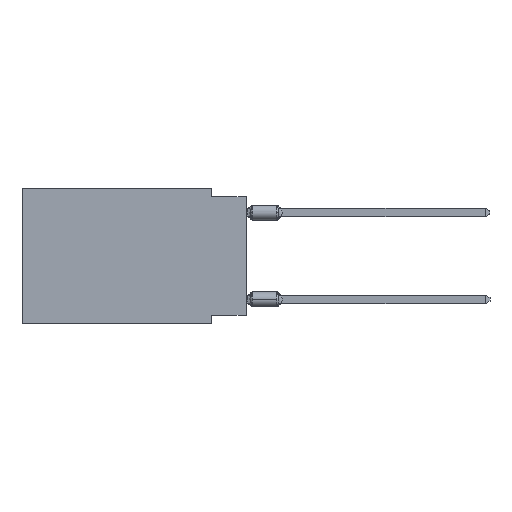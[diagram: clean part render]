
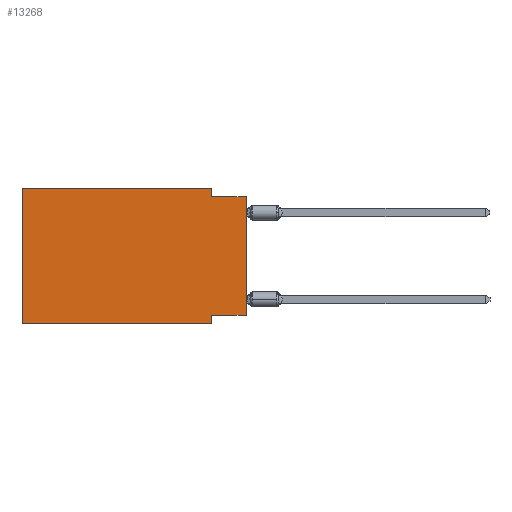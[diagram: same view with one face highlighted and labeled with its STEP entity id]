
A CAD part, left-side view. The second image highlights one B-rep face of the part: STEP entity #13268.
In plain terms, the highlighted planar face has unit normal (-1, 0, 0).
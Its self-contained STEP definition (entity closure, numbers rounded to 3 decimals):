
#137 = LINE ( 'NONE', #13860, #9160 ) ;
#380 = VERTEX_POINT ( 'NONE', #4488 ) ;
#620 = CARTESIAN_POINT ( 'NONE',  ( 0., 16.383, 0. ) ) ;
#703 = DIRECTION ( 'NONE',  ( 0., 0., -1. ) ) ;
#1499 = LINE ( 'NONE', #11670, #16042 ) ;
#1540 = EDGE_LOOP ( 'NONE', ( #11671, #7039, #22111, #13232, #17227, #22080, #11189, #18426 ) ) ;
#2026 = VECTOR ( 'NONE', #18082, 1000. ) ;
#3211 = LINE ( 'NONE', #4708, #3430 ) ;
#3430 = VECTOR ( 'NONE', #10124, 1000. ) ;
#4158 = VERTEX_POINT ( 'NONE', #11063 ) ;
#4194 = DIRECTION ( 'NONE',  ( 0., -1., 0. ) ) ;
#4488 = CARTESIAN_POINT ( 'NONE',  ( 0., 0., -0.635 ) ) ;
#4615 = DIRECTION ( 'NONE',  ( 0., -1., 0. ) ) ;
#4708 = CARTESIAN_POINT ( 'NONE',  ( 0., 0., -9.271 ) ) ;
#4954 = VECTOR ( 'NONE', #703, 1000. ) ;
#5126 = EDGE_CURVE ( 'NONE', #4158, #380, #12950, .T. ) ;
#5306 = VECTOR ( 'NONE', #7950, 1000. ) ;
#5667 = EDGE_CURVE ( 'NONE', #21052, #10206, #1499, .T. ) ;
#6763 = CARTESIAN_POINT ( 'NONE',  ( 0., 2.54, -9.906 ) ) ;
#6931 = DIRECTION ( 'NONE',  ( 0., 0., 1. ) ) ;
#7039 = ORIENTED_EDGE ( 'NONE', *, *, #5126, .F. ) ;
#7735 = FACE_OUTER_BOUND ( 'NONE', #1540, .T. ) ;
#7950 = DIRECTION ( 'NONE',  ( 0., 0., -1. ) ) ;
#8079 = EDGE_CURVE ( 'NONE', #21060, #380, #137, .T. ) ;
#8162 = CARTESIAN_POINT ( 'NONE',  ( 0., 2.54, -9.906 ) ) ;
#8171 = CARTESIAN_POINT ( 'NONE',  ( 0., 0., -9.271 ) ) ;
#8907 = LINE ( 'NONE', #620, #12658 ) ;
#9160 = VECTOR ( 'NONE', #6931, 1000. ) ;
#9628 = CARTESIAN_POINT ( 'NONE',  ( 0., 2.54, 0. ) ) ;
#9960 = EDGE_CURVE ( 'NONE', #21052, #18334, #16240, .T. ) ;
#10124 = DIRECTION ( 'NONE',  ( 0., 1., 0. ) ) ;
#10206 = VERTEX_POINT ( 'NONE', #6763 ) ;
#11063 = CARTESIAN_POINT ( 'NONE',  ( 0., 2.54, -0.635 ) ) ;
#11189 = ORIENTED_EDGE ( 'NONE', *, *, #16235, .F. ) ;
#11263 = CARTESIAN_POINT ( 'NONE',  ( 0., 16.383, 0. ) ) ;
#11670 = CARTESIAN_POINT ( 'NONE',  ( 0., 16.383, -9.906 ) ) ;
#11671 = ORIENTED_EDGE ( 'NONE', *, *, #8079, .T. ) ;
#12658 = VECTOR ( 'NONE', #14438, 1000. ) ;
#12950 = LINE ( 'NONE', #13288, #16389 ) ;
#13178 = DIRECTION ( 'NONE',  ( 0., 0., -1. ) ) ;
#13232 = ORIENTED_EDGE ( 'NONE', *, *, #14227, .F. ) ;
#13268 = ADVANCED_FACE ( 'NONE', ( #7735 ), #19958, .F. ) ;
#13288 = CARTESIAN_POINT ( 'NONE',  ( 0., 0., -0.635 ) ) ;
#13737 = AXIS2_PLACEMENT_3D ( 'NONE', #21693, #16515, #13178 ) ;
#13830 = CARTESIAN_POINT ( 'NONE',  ( 0., 16.383, -9.906 ) ) ;
#13860 = CARTESIAN_POINT ( 'NONE',  ( 0., 0., 0. ) ) ;
#14227 = EDGE_CURVE ( 'NONE', #18334, #18308, #8907, .T. ) ;
#14438 = DIRECTION ( 'NONE',  ( 0., -1., 0. ) ) ;
#14790 = EDGE_CURVE ( 'NONE', #18308, #4158, #16833, .T. ) ;
#16042 = VECTOR ( 'NONE', #4615, 1000. ) ;
#16235 = EDGE_CURVE ( 'NONE', #18089, #10206, #22014, .T. ) ;
#16240 = LINE ( 'NONE', #18209, #2026 ) ;
#16389 = VECTOR ( 'NONE', #4194, 1000. ) ;
#16515 = DIRECTION ( 'NONE',  ( 1., 0., 0. ) ) ;
#16833 = LINE ( 'NONE', #18674, #4954 ) ;
#17227 = ORIENTED_EDGE ( 'NONE', *, *, #9960, .F. ) ;
#18082 = DIRECTION ( 'NONE',  ( 0., 0., 1. ) ) ;
#18089 = VERTEX_POINT ( 'NONE', #20939 ) ;
#18209 = CARTESIAN_POINT ( 'NONE',  ( 0., 16.383, 0. ) ) ;
#18308 = VERTEX_POINT ( 'NONE', #9628 ) ;
#18334 = VERTEX_POINT ( 'NONE', #11263 ) ;
#18426 = ORIENTED_EDGE ( 'NONE', *, *, #21397, .F. ) ;
#18674 = CARTESIAN_POINT ( 'NONE',  ( 0., 2.54, 0. ) ) ;
#19958 = PLANE ( 'NONE',  #13737 ) ;
#20939 = CARTESIAN_POINT ( 'NONE',  ( 0., 2.54, -9.271 ) ) ;
#21052 = VERTEX_POINT ( 'NONE', #13830 ) ;
#21060 = VERTEX_POINT ( 'NONE', #8171 ) ;
#21397 = EDGE_CURVE ( 'NONE', #21060, #18089, #3211, .T. ) ;
#21693 = CARTESIAN_POINT ( 'NONE',  ( 0., 16.383, 0. ) ) ;
#22014 = LINE ( 'NONE', #8162, #5306 ) ;
#22080 = ORIENTED_EDGE ( 'NONE', *, *, #5667, .T. ) ;
#22111 = ORIENTED_EDGE ( 'NONE', *, *, #14790, .F. ) ;
